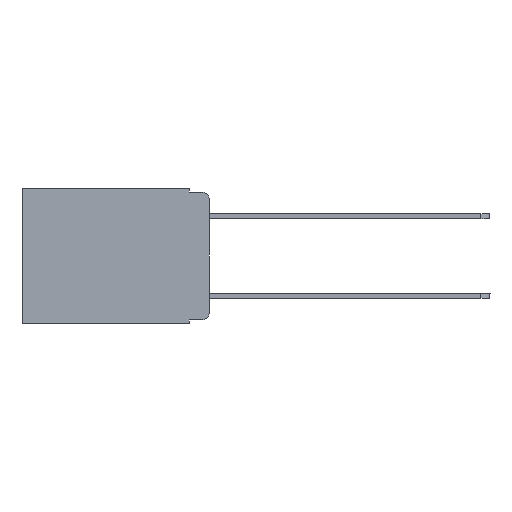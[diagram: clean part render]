
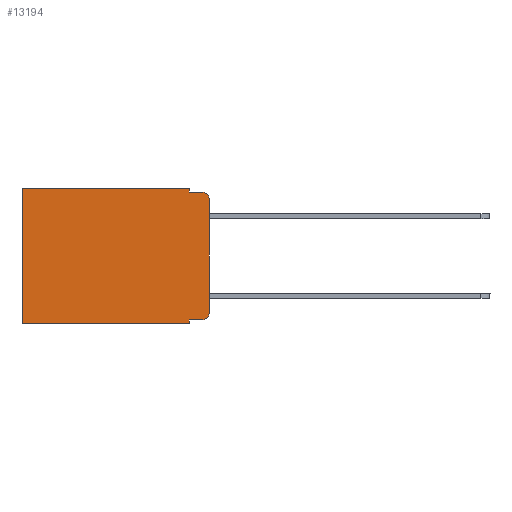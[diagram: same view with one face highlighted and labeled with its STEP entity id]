
A CAD part, left-side view. The second image highlights one B-rep face of the part: STEP entity #13194.
In plain terms, the highlighted planar face has unit normal (-1, 0, 0).
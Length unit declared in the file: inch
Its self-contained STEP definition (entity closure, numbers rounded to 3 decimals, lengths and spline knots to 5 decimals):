
#355 = LINE ( 'NONE', #4485, #15197 ) ;
#550 = ORIENTED_EDGE ( 'NONE', *, *, #3271, .T. ) ;
#950 = VECTOR ( 'NONE', #11128, 39.37008 ) ;
#991 = VERTEX_POINT ( 'NONE', #18922 ) ;
#1253 = DIRECTION ( 'NONE',  ( 0., 0., -1. ) ) ;
#1741 = DIRECTION ( 'NONE',  ( 0., 0., -1. ) ) ;
#1932 = ORIENTED_EDGE ( 'NONE', *, *, #6065, .T. ) ;
#2095 = DIRECTION ( 'NONE',  ( 0., -1., 0. ) ) ;
#2123 = CIRCLE ( 'NONE', #9679, 0.02 ) ;
#2248 = EDGE_CURVE ( 'NONE', #17827, #18730, #19157, .T. ) ;
#2292 = VECTOR ( 'NONE', #1253, 39.37008 ) ;
#2334 = CARTESIAN_POINT ( 'NONE',  ( 0.298, 0.051, -0.343 ) ) ;
#2454 = VERTEX_POINT ( 'NONE', #6919 ) ;
#2705 = VERTEX_POINT ( 'NONE', #15182 ) ;
#3271 = EDGE_CURVE ( 'NONE', #16056, #2705, #2123, .T. ) ;
#3311 = DIRECTION ( 'NONE',  ( -1., 0., 0. ) ) ;
#3414 = VERTEX_POINT ( 'NONE', #15836 ) ;
#4269 = VECTOR ( 'NONE', #8937, 39.37008 ) ;
#4485 = CARTESIAN_POINT ( 'NONE',  ( 0.298, 0., -0.343 ) ) ;
#4706 = VERTEX_POINT ( 'NONE', #2334 ) ;
#4802 = VECTOR ( 'NONE', #2095, 39.37008 ) ;
#4993 = EDGE_CURVE ( 'NONE', #6243, #17414, #10890, .T. ) ;
#5881 = LINE ( 'NONE', #16503, #2292 ) ;
#6053 = AXIS2_PLACEMENT_3D ( 'NONE', #15225, #3311, #6168 ) ;
#6065 = EDGE_CURVE ( 'NONE', #17827, #6243, #6714, .T. ) ;
#6168 = DIRECTION ( 'NONE',  ( 0., 0., -1. ) ) ;
#6243 = VERTEX_POINT ( 'NONE', #16825 ) ;
#6714 = LINE ( 'NONE', #18699, #18775 ) ;
#6919 = CARTESIAN_POINT ( 'NONE',  ( 0.298, 0.02, -0.01 ) ) ;
#7110 = ORIENTED_EDGE ( 'NONE', *, *, #12596, .F. ) ;
#7375 = ORIENTED_EDGE ( 'NONE', *, *, #15939, .T. ) ;
#7632 = CIRCLE ( 'NONE', #6053, 0.02 ) ;
#7824 = CARTESIAN_POINT ( 'NONE',  ( 0.298, 0.051, -0.01 ) ) ;
#8606 = VECTOR ( 'NONE', #13693, 39.37008 ) ;
#8693 = EDGE_CURVE ( 'NONE', #3414, #4706, #14389, .T. ) ;
#8937 = DIRECTION ( 'NONE',  ( 0., 0., -1. ) ) ;
#9148 = ORIENTED_EDGE ( 'NONE', *, *, #2248, .F. ) ;
#9170 = LINE ( 'NONE', #10922, #8606 ) ;
#9326 = DIRECTION ( 'NONE',  ( 0., 1., 0. ) ) ;
#9449 = DIRECTION ( 'NONE',  ( -1., 0., 0. ) ) ;
#9537 = CARTESIAN_POINT ( 'NONE',  ( 0.298, 0.02, -0.313 ) ) ;
#9574 = ORIENTED_EDGE ( 'NONE', *, *, #14682, .F. ) ;
#9679 = AXIS2_PLACEMENT_3D ( 'NONE', #9537, #9449, #15551 ) ;
#9959 = CARTESIAN_POINT ( 'NONE',  ( 0.298, 0.051, 0. ) ) ;
#10890 = LINE ( 'NONE', #12266, #15617 ) ;
#10922 = CARTESIAN_POINT ( 'NONE',  ( 0.298, 0.051, -0.333 ) ) ;
#11128 = DIRECTION ( 'NONE',  ( 0., 0., -1. ) ) ;
#11307 = ORIENTED_EDGE ( 'NONE', *, *, #4993, .T. ) ;
#11517 = PLANE ( 'NONE',  #15517 ) ;
#11681 = ORIENTED_EDGE ( 'NONE', *, *, #15127, .T. ) ;
#12266 = CARTESIAN_POINT ( 'NONE',  ( 0.298, 0.473, 0. ) ) ;
#12596 = EDGE_CURVE ( 'NONE', #18730, #2454, #15014, .T. ) ;
#12613 = CARTESIAN_POINT ( 'NONE',  ( 0.298, 0.051, 0. ) ) ;
#12695 = DIRECTION ( 'NONE',  ( 0., 1., 0. ) ) ;
#12924 = CARTESIAN_POINT ( 'NONE',  ( 0.298, 0.473, -0.343 ) ) ;
#12979 = CARTESIAN_POINT ( 'NONE',  ( 0.298, 0., 0. ) ) ;
#13086 = FACE_OUTER_BOUND ( 'NONE', #16618, .T. ) ;
#13194 = ADVANCED_FACE ( 'NONE', ( #13086 ), #11517, .F. ) ;
#13693 = DIRECTION ( 'NONE',  ( 0., -1., 0. ) ) ;
#14389 = LINE ( 'NONE', #9959, #950 ) ;
#14682 = EDGE_CURVE ( 'NONE', #4706, #17414, #355, .T. ) ;
#15002 = ORIENTED_EDGE ( 'NONE', *, *, #17076, .F. ) ;
#15014 = LINE ( 'NONE', #15408, #4802 ) ;
#15127 = EDGE_CURVE ( 'NONE', #3414, #16056, #9170, .T. ) ;
#15182 = CARTESIAN_POINT ( 'NONE',  ( 0.298, 0., -0.313 ) ) ;
#15197 = VECTOR ( 'NONE', #9326, 39.37008 ) ;
#15225 = CARTESIAN_POINT ( 'NONE',  ( 0.298, 0.02, -0.03 ) ) ;
#15408 = CARTESIAN_POINT ( 'NONE',  ( 0.298, 0.051, -0.01 ) ) ;
#15469 = ORIENTED_EDGE ( 'NONE', *, *, #8693, .F. ) ;
#15517 = AXIS2_PLACEMENT_3D ( 'NONE', #12979, #19089, #17534 ) ;
#15551 = DIRECTION ( 'NONE',  ( 0., 0., -1. ) ) ;
#15617 = VECTOR ( 'NONE', #1741, 39.37008 ) ;
#15836 = CARTESIAN_POINT ( 'NONE',  ( 0.298, 0.051, -0.333 ) ) ;
#15939 = EDGE_CURVE ( 'NONE', #991, #2454, #7632, .T. ) ;
#16056 = VERTEX_POINT ( 'NONE', #17000 ) ;
#16408 = CARTESIAN_POINT ( 'NONE',  ( 0.298, 0.051, 0. ) ) ;
#16503 = CARTESIAN_POINT ( 'NONE',  ( 0.298, 0., 0. ) ) ;
#16618 = EDGE_LOOP ( 'NONE', ( #15002, #7375, #7110, #9148, #1932, #11307, #9574, #15469, #11681, #550 ) ) ;
#16825 = CARTESIAN_POINT ( 'NONE',  ( 0.298, 0.473, 0. ) ) ;
#17000 = CARTESIAN_POINT ( 'NONE',  ( 0.298, 0.02, -0.333 ) ) ;
#17076 = EDGE_CURVE ( 'NONE', #991, #2705, #5881, .T. ) ;
#17414 = VERTEX_POINT ( 'NONE', #12924 ) ;
#17534 = DIRECTION ( 'NONE',  ( 0., 0., -1. ) ) ;
#17827 = VERTEX_POINT ( 'NONE', #12613 ) ;
#18699 = CARTESIAN_POINT ( 'NONE',  ( 0.298, 0., 0. ) ) ;
#18730 = VERTEX_POINT ( 'NONE', #7824 ) ;
#18775 = VECTOR ( 'NONE', #12695, 39.37008 ) ;
#18922 = CARTESIAN_POINT ( 'NONE',  ( 0.298, 0., -0.03 ) ) ;
#19089 = DIRECTION ( 'NONE',  ( 1., 0., 0. ) ) ;
#19157 = LINE ( 'NONE', #16408, #4269 ) ;
